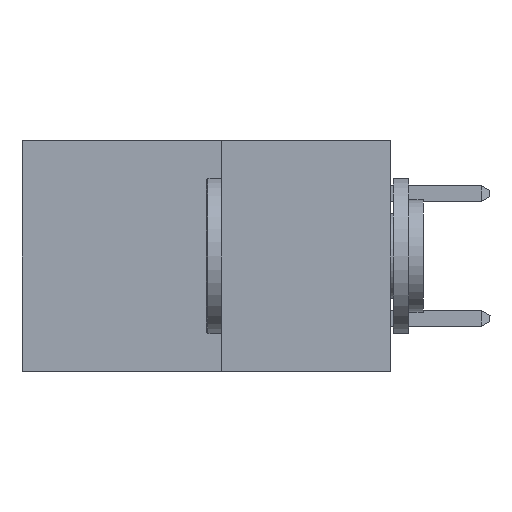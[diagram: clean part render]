
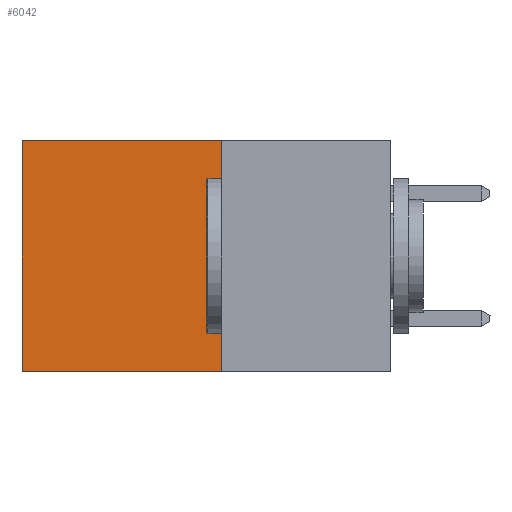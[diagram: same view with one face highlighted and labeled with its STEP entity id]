
A CAD part, left-side view. The second image highlights one B-rep face of the part: STEP entity #6042.
In plain terms, the highlighted planar face has unit normal (-1, 0, 0).
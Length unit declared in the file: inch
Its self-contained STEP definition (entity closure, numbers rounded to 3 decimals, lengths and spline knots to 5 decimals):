
#2231 = VECTOR ( 'NONE', #31550, 39.37008 ) ;
#2327 = DIRECTION ( 'NONE',  ( 0., 1., 0. ) ) ;
#2372 = VERTEX_POINT ( 'NONE', #6695 ) ;
#3700 = EDGE_LOOP ( 'NONE', ( #11573, #26465, #23621, #24647 ) ) ;
#3974 = EDGE_CURVE ( 'NONE', #22609, #28004, #19239, .T. ) ;
#4922 = CARTESIAN_POINT ( 'NONE',  ( 0.277, 0.59, -0.37 ) ) ;
#6042 = ADVANCED_FACE ( 'NONE', ( #26043 ), #22860, .F. ) ;
#6179 = CARTESIAN_POINT ( 'NONE',  ( 0.277, 0.27, 0. ) ) ;
#6228 = LINE ( 'NONE', #9024, #31782 ) ;
#6695 = CARTESIAN_POINT ( 'NONE',  ( 0.277, 0.59, 0. ) ) ;
#9024 = CARTESIAN_POINT ( 'NONE',  ( 0.277, 0.59, -0.37 ) ) ;
#9717 = DIRECTION ( 'NONE',  ( 0., 1., 0. ) ) ;
#9727 = LINE ( 'NONE', #26663, #2231 ) ;
#10503 = EDGE_CURVE ( 'NONE', #2372, #28004, #6228, .T. ) ;
#11232 = CARTESIAN_POINT ( 'NONE',  ( 0.277, 0.27, -0.37 ) ) ;
#11436 = EDGE_CURVE ( 'NONE', #30655, #2372, #30955, .T. ) ;
#11573 = ORIENTED_EDGE ( 'NONE', *, *, #10503, .T. ) ;
#16491 = DIRECTION ( 'NONE',  ( 0., 0., -1. ) ) ;
#17303 = CARTESIAN_POINT ( 'NONE',  ( 0.277, 0.27, 0. ) ) ;
#18649 = VECTOR ( 'NONE', #2327, 39.37008 ) ;
#19239 = LINE ( 'NONE', #11232, #25794 ) ;
#19740 = AXIS2_PLACEMENT_3D ( 'NONE', #22789, #22971, #22753 ) ;
#22609 = VERTEX_POINT ( 'NONE', #32125 ) ;
#22753 = DIRECTION ( 'NONE',  ( 0., 0., -1. ) ) ;
#22789 = CARTESIAN_POINT ( 'NONE',  ( 0.277, 0.27, -0.37 ) ) ;
#22860 = PLANE ( 'NONE',  #19740 ) ;
#22971 = DIRECTION ( 'NONE',  ( 1., 0., 0. ) ) ;
#23621 = ORIENTED_EDGE ( 'NONE', *, *, #31498, .F. ) ;
#24647 = ORIENTED_EDGE ( 'NONE', *, *, #11436, .T. ) ;
#25794 = VECTOR ( 'NONE', #9717, 39.37008 ) ;
#26043 = FACE_OUTER_BOUND ( 'NONE', #3700, .T. ) ;
#26465 = ORIENTED_EDGE ( 'NONE', *, *, #3974, .F. ) ;
#26663 = CARTESIAN_POINT ( 'NONE',  ( 0.277, 0.27, -0.37 ) ) ;
#28004 = VERTEX_POINT ( 'NONE', #4922 ) ;
#30655 = VERTEX_POINT ( 'NONE', #6179 ) ;
#30955 = LINE ( 'NONE', #17303, #18649 ) ;
#31498 = EDGE_CURVE ( 'NONE', #30655, #22609, #9727, .T. ) ;
#31550 = DIRECTION ( 'NONE',  ( 0., 0., -1. ) ) ;
#31782 = VECTOR ( 'NONE', #16491, 39.37008 ) ;
#32125 = CARTESIAN_POINT ( 'NONE',  ( 0.277, 0.27, -0.37 ) ) ;
